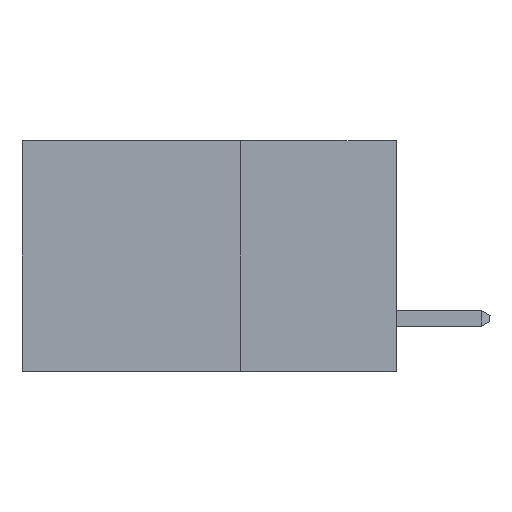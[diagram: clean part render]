
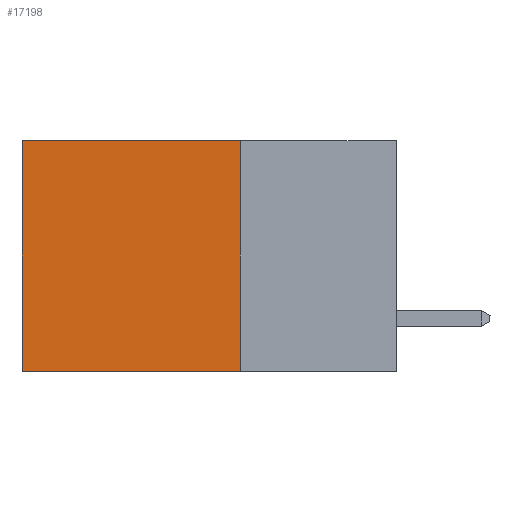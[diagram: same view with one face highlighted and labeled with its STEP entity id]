
A CAD part, left-side view. The second image highlights one B-rep face of the part: STEP entity #17198.
In plain terms, the highlighted planar face has unit normal (-1, 0, 0).
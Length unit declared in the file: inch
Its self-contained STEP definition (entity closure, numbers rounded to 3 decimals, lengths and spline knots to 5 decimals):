
#16 = VECTOR ( 'NONE', #7746, 39.37008 ) ;
#520 = VERTEX_POINT ( 'NONE', #10475 ) ;
#1075 = PLANE ( 'NONE',  #2234 ) ;
#1838 = VERTEX_POINT ( 'NONE', #13059 ) ;
#1920 = EDGE_CURVE ( 'NONE', #520, #10658, #12003, .T. ) ;
#2229 = CARTESIAN_POINT ( 'NONE',  ( 0.298, 0.6, 0. ) ) ;
#2234 = AXIS2_PLACEMENT_3D ( 'NONE', #2634, #16343, #2452 ) ;
#2452 = DIRECTION ( 'NONE',  ( 0., 0., -1. ) ) ;
#2634 = CARTESIAN_POINT ( 'NONE',  ( 0.298, 0.25, 0. ) ) ;
#2835 = CARTESIAN_POINT ( 'NONE',  ( 0.298, 0.25, 0. ) ) ;
#3301 = ORIENTED_EDGE ( 'NONE', *, *, #10934, .T. ) ;
#4340 = EDGE_LOOP ( 'NONE', ( #14382, #6568, #4697, #3301 ) ) ;
#4697 = ORIENTED_EDGE ( 'NONE', *, *, #10505, .F. ) ;
#6438 = VECTOR ( 'NONE', #8440, 39.37008 ) ;
#6568 = ORIENTED_EDGE ( 'NONE', *, *, #1920, .F. ) ;
#7184 = VECTOR ( 'NONE', #15321, 39.37008 ) ;
#7746 = DIRECTION ( 'NONE',  ( 0., 0., -1. ) ) ;
#8200 = CARTESIAN_POINT ( 'NONE',  ( 0.298, 0.25, -0.37 ) ) ;
#8440 = DIRECTION ( 'NONE',  ( 0., 1., 0. ) ) ;
#8751 = LINE ( 'NONE', #2229, #16 ) ;
#8929 = CARTESIAN_POINT ( 'NONE',  ( 0.298, 0.25, 0. ) ) ;
#10475 = CARTESIAN_POINT ( 'NONE',  ( 0.298, 0.25, -0.37 ) ) ;
#10505 = EDGE_CURVE ( 'NONE', #17401, #520, #14934, .T. ) ;
#10658 = VERTEX_POINT ( 'NONE', #12167 ) ;
#10826 = LINE ( 'NONE', #15431, #7184 ) ;
#10934 = EDGE_CURVE ( 'NONE', #17401, #1838, #10826, .T. ) ;
#11898 = VECTOR ( 'NONE', #17181, 39.37008 ) ;
#12003 = LINE ( 'NONE', #8200, #6438 ) ;
#12167 = CARTESIAN_POINT ( 'NONE',  ( 0.298, 0.6, -0.37 ) ) ;
#12903 = FACE_OUTER_BOUND ( 'NONE', #4340, .T. ) ;
#13059 = CARTESIAN_POINT ( 'NONE',  ( 0.298, 0.6, 0. ) ) ;
#13823 = EDGE_CURVE ( 'NONE', #1838, #10658, #8751, .T. ) ;
#14382 = ORIENTED_EDGE ( 'NONE', *, *, #13823, .T. ) ;
#14934 = LINE ( 'NONE', #8929, #11898 ) ;
#15321 = DIRECTION ( 'NONE',  ( 0., 1., 0. ) ) ;
#15431 = CARTESIAN_POINT ( 'NONE',  ( 0.298, 0.25, 0. ) ) ;
#16343 = DIRECTION ( 'NONE',  ( 1., 0., 0. ) ) ;
#17181 = DIRECTION ( 'NONE',  ( 0., 0., -1. ) ) ;
#17198 = ADVANCED_FACE ( 'NONE', ( #12903 ), #1075, .F. ) ;
#17401 = VERTEX_POINT ( 'NONE', #2835 ) ;
